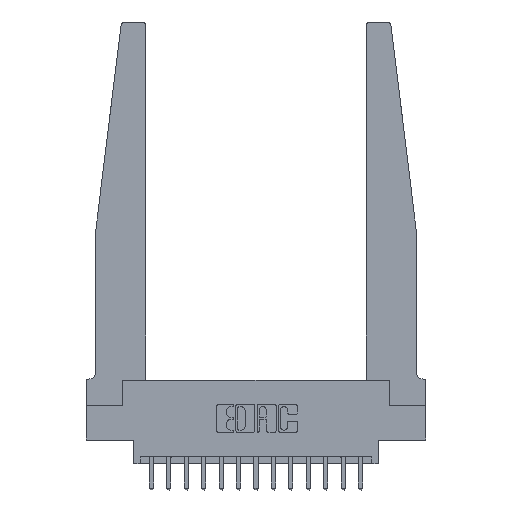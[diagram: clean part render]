
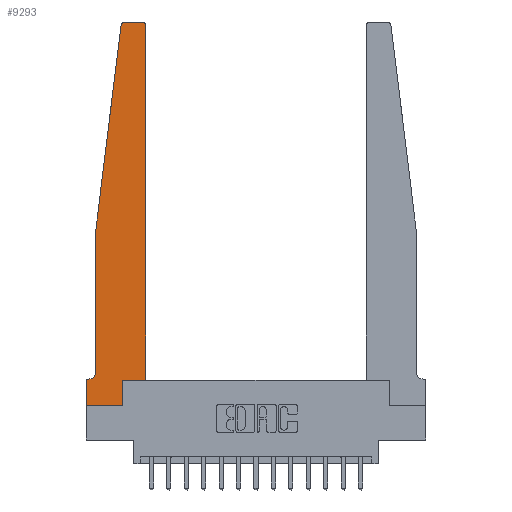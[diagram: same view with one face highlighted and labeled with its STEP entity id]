
A CAD part, top view. The second image highlights one B-rep face of the part: STEP entity #9293.
In plain terms, the highlighted planar face has unit normal (0, 0, 1).
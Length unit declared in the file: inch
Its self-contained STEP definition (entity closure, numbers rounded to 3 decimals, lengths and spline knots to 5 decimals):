
#57 = CARTESIAN_POINT ( 'NONE',  ( 0., 0.1875, 0.37 ) ) ;
#356 = DIRECTION ( 'NONE',  ( 0., 0., -1. ) ) ;
#410 = CARTESIAN_POINT ( 'NONE',  ( 0.065, 0.2375, 0.37 ) ) ;
#442 = VERTEX_POINT ( 'NONE', #410 ) ;
#629 = VERTEX_POINT ( 'NONE', #1321 ) ;
#685 = CARTESIAN_POINT ( 'NONE',  ( 0.27653, 2.75, 0.37 ) ) ;
#687 = CARTESIAN_POINT ( 'NONE',  ( 0., 0.1875, 0.37 ) ) ;
#696 = ORIENTED_EDGE ( 'NONE', *, *, #17317, .T. ) ;
#739 = VECTOR ( 'NONE', #12679, 39.37008 ) ;
#775 = PLANE ( 'NONE',  #5888 ) ;
#796 = DIRECTION ( 'NONE',  ( 0., 1., 0. ) ) ;
#855 = EDGE_LOOP ( 'NONE', ( #11627, #13525, #3607, #5507, #9858, #15234, #16633, #6137, #5848, #12062, #16879, #696 ) ) ;
#1321 = CARTESIAN_POINT ( 'NONE',  ( 0.24675, 2.72367, 0.37 ) ) ;
#1332 = EDGE_CURVE ( 'NONE', #14081, #16752, #1561, .T. ) ;
#1561 = LINE ( 'NONE', #1644, #4317 ) ;
#1567 = DIRECTION ( 'NONE',  ( 1., 0., 0. ) ) ;
#1644 = CARTESIAN_POINT ( 'NONE',  ( 0.065, 0.1875, 0.37 ) ) ;
#2039 = FACE_OUTER_BOUND ( 'NONE', #855, .T. ) ;
#2113 = VERTEX_POINT ( 'NONE', #14030 ) ;
#2256 = VECTOR ( 'NONE', #17792, 39.37008 ) ;
#2770 = CARTESIAN_POINT ( 'NONE',  ( 0.425, 2.72, 0.37 ) ) ;
#2854 = VERTEX_POINT ( 'NONE', #4889 ) ;
#2995 = AXIS2_PLACEMENT_3D ( 'NONE', #8930, #12981, #3809 ) ;
#3304 = DIRECTION ( 'NONE',  ( 1., 0., 0. ) ) ;
#3407 = CARTESIAN_POINT ( 'NONE',  ( 0.2605, 0.18, 0.37 ) ) ;
#3475 = DIRECTION ( 'NONE',  ( 0., 0., 1. ) ) ;
#3607 = ORIENTED_EDGE ( 'NONE', *, *, #14697, .T. ) ;
#3695 = VECTOR ( 'NONE', #14750, 39.37008 ) ;
#3809 = DIRECTION ( 'NONE',  ( 1., 0., 0. ) ) ;
#4277 = DIRECTION ( 'NONE',  ( -1., 0., 0. ) ) ;
#4317 = VECTOR ( 'NONE', #4277, 39.37008 ) ;
#4422 = AXIS2_PLACEMENT_3D ( 'NONE', #8761, #356, #7217 ) ;
#4651 = CARTESIAN_POINT ( 'NONE',  ( 0.395, 2.72, 0.37 ) ) ;
#4788 = VECTOR ( 'NONE', #1567, 39.37008 ) ;
#4846 = DIRECTION ( 'NONE',  ( 1., 0., 0. ) ) ;
#4889 = CARTESIAN_POINT ( 'NONE',  ( 0.065, 1.25, 0.37 ) ) ;
#5029 = CIRCLE ( 'NONE', #2995, 0.03 ) ;
#5131 = VERTEX_POINT ( 'NONE', #2770 ) ;
#5377 = VECTOR ( 'NONE', #10921, 39.37008 ) ;
#5507 = ORIENTED_EDGE ( 'NONE', *, *, #10668, .T. ) ;
#5580 = VECTOR ( 'NONE', #10278, 39.37008 ) ;
#5848 = ORIENTED_EDGE ( 'NONE', *, *, #8902, .T. ) ;
#5888 = AXIS2_PLACEMENT_3D ( 'NONE', #687, #10406, #4846 ) ;
#5929 = VERTEX_POINT ( 'NONE', #685 ) ;
#6116 = CIRCLE ( 'NONE', #16225, 0.03 ) ;
#6137 = ORIENTED_EDGE ( 'NONE', *, *, #11592, .T. ) ;
#6606 = VERTEX_POINT ( 'NONE', #15024 ) ;
#7217 = DIRECTION ( 'NONE',  ( -1., 0., 0. ) ) ;
#8054 = LINE ( 'NONE', #9239, #3695 ) ;
#8196 = EDGE_CURVE ( 'NONE', #442, #14081, #9878, .T. ) ;
#8290 = EDGE_CURVE ( 'NONE', #5929, #629, #5029, .T. ) ;
#8303 = EDGE_CURVE ( 'NONE', #16752, #16980, #9296, .T. ) ;
#8394 = LINE ( 'NONE', #9573, #5377 ) ;
#8545 = CARTESIAN_POINT ( 'NONE',  ( 0.065, 1.25, 0.37 ) ) ;
#8761 = CARTESIAN_POINT ( 'NONE',  ( 0.015, 0.2375, 0.37 ) ) ;
#8902 = EDGE_CURVE ( 'NONE', #10215, #9848, #9184, .T. ) ;
#8930 = CARTESIAN_POINT ( 'NONE',  ( 0.27653, 2.72, 0.37 ) ) ;
#9025 = CARTESIAN_POINT ( 'NONE',  ( 0., 0., 0.37 ) ) ;
#9184 = LINE ( 'NONE', #13344, #11943 ) ;
#9239 = CARTESIAN_POINT ( 'NONE',  ( 0.065, 1.25, 0.37 ) ) ;
#9293 = ADVANCED_FACE ( 'NONE', ( #2039 ), #775, .T. ) ;
#9296 = LINE ( 'NONE', #9025, #5580 ) ;
#9492 = LINE ( 'NONE', #15003, #2256 ) ;
#9573 = CARTESIAN_POINT ( 'NONE',  ( 0.425, 0.18, 0.37 ) ) ;
#9589 = DIRECTION ( 'NONE',  ( -1., 0., 0. ) ) ;
#9759 = CARTESIAN_POINT ( 'NONE',  ( 0., 0., 0.37 ) ) ;
#9848 = VERTEX_POINT ( 'NONE', #3407 ) ;
#9858 = ORIENTED_EDGE ( 'NONE', *, *, #8196, .T. ) ;
#9878 = CIRCLE ( 'NONE', #4422, 0.05 ) ;
#10056 = CARTESIAN_POINT ( 'NONE',  ( 0., 0., 0.37 ) ) ;
#10215 = VERTEX_POINT ( 'NONE', #13492 ) ;
#10278 = DIRECTION ( 'NONE',  ( 0., -1., 0. ) ) ;
#10406 = DIRECTION ( 'NONE',  ( 0., 0., 1. ) ) ;
#10510 = CARTESIAN_POINT ( 'NONE',  ( 0.015, 0.1875, 0.37 ) ) ;
#10668 = EDGE_CURVE ( 'NONE', #2854, #442, #10739, .T. ) ;
#10739 = LINE ( 'NONE', #8545, #739 ) ;
#10921 = DIRECTION ( 'NONE',  ( 0., 1., 0. ) ) ;
#11527 = VECTOR ( 'NONE', #9589, 39.37008 ) ;
#11592 = EDGE_CURVE ( 'NONE', #16980, #10215, #16471, .T. ) ;
#11627 = ORIENTED_EDGE ( 'NONE', *, *, #15748, .T. ) ;
#11943 = VECTOR ( 'NONE', #796, 39.37008 ) ;
#12034 = EDGE_CURVE ( 'NONE', #2113, #5131, #8394, .T. ) ;
#12062 = ORIENTED_EDGE ( 'NONE', *, *, #13141, .T. ) ;
#12679 = DIRECTION ( 'NONE',  ( 0., -1., 0. ) ) ;
#12981 = DIRECTION ( 'NONE',  ( 0., 0., 1. ) ) ;
#13141 = EDGE_CURVE ( 'NONE', #9848, #2113, #9492, .T. ) ;
#13344 = CARTESIAN_POINT ( 'NONE',  ( 0.2605, 0.18, 0.37 ) ) ;
#13492 = CARTESIAN_POINT ( 'NONE',  ( 0.2605, 0., 0.37 ) ) ;
#13525 = ORIENTED_EDGE ( 'NONE', *, *, #8290, .T. ) ;
#13671 = LINE ( 'NONE', #17806, #11527 ) ;
#14030 = CARTESIAN_POINT ( 'NONE',  ( 0.425, 0.18, 0.37 ) ) ;
#14081 = VERTEX_POINT ( 'NONE', #10510 ) ;
#14697 = EDGE_CURVE ( 'NONE', #629, #2854, #8054, .T. ) ;
#14750 = DIRECTION ( 'NONE',  ( -0.122, -0.992, 0. ) ) ;
#15003 = CARTESIAN_POINT ( 'NONE',  ( 0.425, 0.18, 0.37 ) ) ;
#15024 = CARTESIAN_POINT ( 'NONE',  ( 0.395, 2.75, 0.37 ) ) ;
#15234 = ORIENTED_EDGE ( 'NONE', *, *, #1332, .T. ) ;
#15748 = EDGE_CURVE ( 'NONE', #6606, #5929, #13671, .T. ) ;
#16225 = AXIS2_PLACEMENT_3D ( 'NONE', #4651, #3475, #3304 ) ;
#16471 = LINE ( 'NONE', #9759, #4788 ) ;
#16633 = ORIENTED_EDGE ( 'NONE', *, *, #8303, .T. ) ;
#16752 = VERTEX_POINT ( 'NONE', #57 ) ;
#16879 = ORIENTED_EDGE ( 'NONE', *, *, #12034, .T. ) ;
#16980 = VERTEX_POINT ( 'NONE', #10056 ) ;
#17317 = EDGE_CURVE ( 'NONE', #5131, #6606, #6116, .T. ) ;
#17792 = DIRECTION ( 'NONE',  ( 1., 0., 0. ) ) ;
#17806 = CARTESIAN_POINT ( 'NONE',  ( 0.25, 2.75, 0.37 ) ) ;
